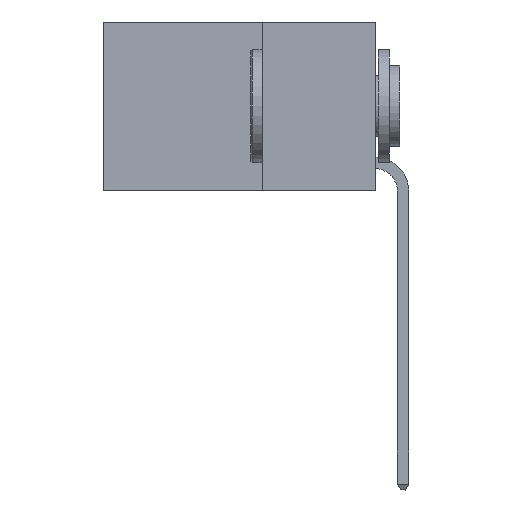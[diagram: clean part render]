
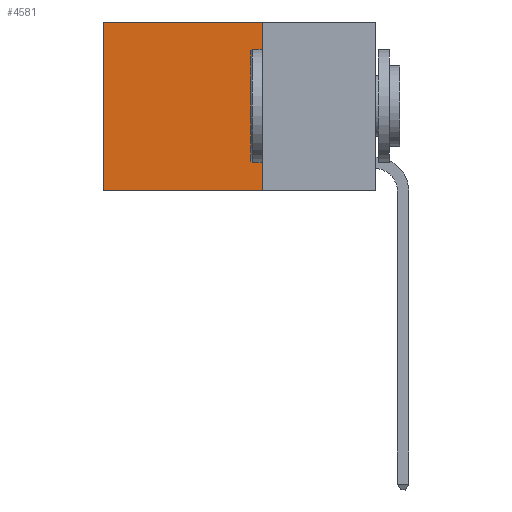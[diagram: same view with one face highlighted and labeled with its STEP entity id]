
A CAD part, left-side view. The second image highlights one B-rep face of the part: STEP entity #4581.
In plain terms, the highlighted planar face has unit normal (-1, 0, 0).
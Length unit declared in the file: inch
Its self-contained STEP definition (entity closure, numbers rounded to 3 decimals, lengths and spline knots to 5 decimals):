
#69 = LINE ( 'NONE', #7998, #11760 ) ;
#464 = ORIENTED_EDGE ( 'NONE', *, *, #581, .T. ) ;
#581 = EDGE_CURVE ( 'NONE', #12068, #16119, #16625, .T. ) ;
#2050 = CARTESIAN_POINT ( 'NONE',  ( 0.2625, 0.25, 0. ) ) ;
#2405 = VERTEX_POINT ( 'NONE', #21548 ) ;
#3027 = LINE ( 'NONE', #22992, #12869 ) ;
#4309 = DIRECTION ( 'NONE',  ( 0., 0., -1. ) ) ;
#4581 = ADVANCED_FACE ( 'NONE', ( #9815 ), #22323, .F. ) ;
#5135 = ORIENTED_EDGE ( 'NONE', *, *, #18441, .F. ) ;
#6088 = CARTESIAN_POINT ( 'NONE',  ( 0.2625, 0.25, 0. ) ) ;
#7047 = CARTESIAN_POINT ( 'NONE',  ( 0.2625, 0.6, -0.37 ) ) ;
#7763 = EDGE_CURVE ( 'NONE', #2405, #8970, #3027, .T. ) ;
#7781 = DIRECTION ( 'NONE',  ( 0., 0., -1. ) ) ;
#7998 = CARTESIAN_POINT ( 'NONE',  ( 0.2625, 0.6, 0. ) ) ;
#8970 = VERTEX_POINT ( 'NONE', #7047 ) ;
#9815 = FACE_OUTER_BOUND ( 'NONE', #23453, .T. ) ;
#11410 = CARTESIAN_POINT ( 'NONE',  ( 0.2625, 0.25, 0. ) ) ;
#11760 = VECTOR ( 'NONE', #4309, 39.37008 ) ;
#12067 = DIRECTION ( 'NONE',  ( 0., 1., 0. ) ) ;
#12068 = VERTEX_POINT ( 'NONE', #6088 ) ;
#12330 = VECTOR ( 'NONE', #13020, 39.37008 ) ;
#12869 = VECTOR ( 'NONE', #12067, 39.37008 ) ;
#13020 = DIRECTION ( 'NONE',  ( 0., 1., 0. ) ) ;
#16119 = VERTEX_POINT ( 'NONE', #16538 ) ;
#16538 = CARTESIAN_POINT ( 'NONE',  ( 0.2625, 0.6, 0. ) ) ;
#16625 = LINE ( 'NONE', #23904, #12330 ) ;
#16968 = VECTOR ( 'NONE', #20523, 39.37008 ) ;
#17539 = LINE ( 'NONE', #2050, #16968 ) ;
#18441 = EDGE_CURVE ( 'NONE', #12068, #2405, #17539, .T. ) ;
#18783 = DIRECTION ( 'NONE',  ( 1., 0., 0. ) ) ;
#19845 = ORIENTED_EDGE ( 'NONE', *, *, #20483, .T. ) ;
#20286 = AXIS2_PLACEMENT_3D ( 'NONE', #11410, #18783, #7781 ) ;
#20483 = EDGE_CURVE ( 'NONE', #16119, #8970, #69, .T. ) ;
#20523 = DIRECTION ( 'NONE',  ( 0., 0., -1. ) ) ;
#21548 = CARTESIAN_POINT ( 'NONE',  ( 0.2625, 0.25, -0.37 ) ) ;
#21653 = ORIENTED_EDGE ( 'NONE', *, *, #7763, .F. ) ;
#22323 = PLANE ( 'NONE',  #20286 ) ;
#22992 = CARTESIAN_POINT ( 'NONE',  ( 0.2625, 0.25, -0.37 ) ) ;
#23453 = EDGE_LOOP ( 'NONE', ( #19845, #21653, #5135, #464 ) ) ;
#23904 = CARTESIAN_POINT ( 'NONE',  ( 0.2625, 0.25, 0. ) ) ;
